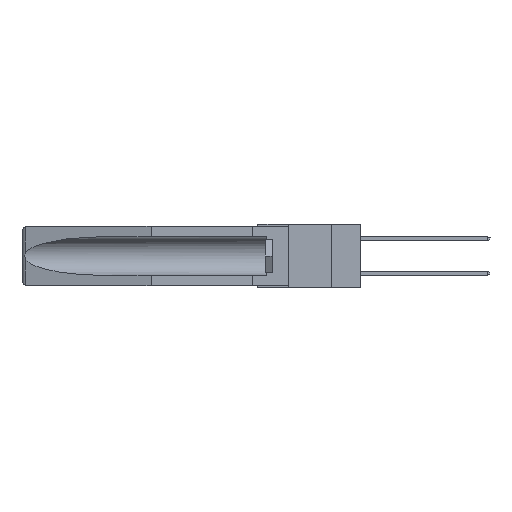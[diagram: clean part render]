
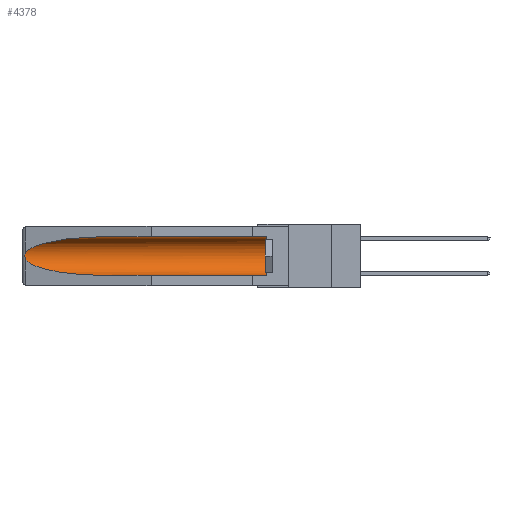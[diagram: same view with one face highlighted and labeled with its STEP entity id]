
A CAD part, left-side view. The second image highlights one B-rep face of the part: STEP entity #4378.
In plain terms, the highlighted cylindrical face has radius 2.857 mm (diameter 5.715 mm), a partial arc.
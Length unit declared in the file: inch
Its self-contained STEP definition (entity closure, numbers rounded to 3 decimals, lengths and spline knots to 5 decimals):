
#299 = EDGE_CURVE ( 'NONE', #5602, #23716, #3488, .T. ) ;
#722 = CARTESIAN_POINT ( 'NONE',  ( 0.155, 1.07973, -0.284 ) ) ;
#1227 = CARTESIAN_POINT ( 'NONE',  ( 0.25451, 1.48313, -0.09465 ) ) ;
#1373 = CARTESIAN_POINT ( 'NONE',  ( 0.155, 0.126, -0.1715 ) ) ;
#1454 = VECTOR ( 'NONE', #25289, 39.37008 ) ;
#3338 = ORIENTED_EDGE ( 'NONE', *, *, #299, .T. ) ;
#3488 = CIRCLE ( 'NONE', #10674, 0.1125 ) ;
#4350 = CARTESIAN_POINT ( 'NONE',  ( 0.25451, 1.48313, -0.24835 ) ) ;
#4378 = ADVANCED_FACE ( 'NONE', ( #20549 ), #23353, .F. ) ;
#4479 = EDGE_LOOP ( 'NONE', ( #23887, #13924, #23803, #11658, #3338, #22921 ) ) ;
#4938 = CARTESIAN_POINT ( 'NONE',  ( 0.155, -0.30754, -0.284 ) ) ;
#5281 = LINE ( 'NONE', #4938, #1454 ) ;
#5602 = VERTEX_POINT ( 'NONE', #13112 ) ;
#7306 = CARTESIAN_POINT ( 'NONE',  ( 0.155, 0.126, -0.059 ) ) ;
#7563 = CARTESIAN_POINT ( 'NONE',  ( 0.2675, 1.53308, -0.17534 ) ) ;
#7994 = CARTESIAN_POINT ( 'NONE',  ( 0.26537, 1.52718, -0.14972 ) ) ;
#9085 = CARTESIAN_POINT ( 'NONE',  ( 0.155, -0.30754, -0.059 ) ) ;
#9726 = CARTESIAN_POINT ( 'NONE',  ( 0.26654, 1.53092, -0.15636 ) ) ;
#10370 = CARTESIAN_POINT ( 'NONE',  ( 0.26537, 1.52718, -0.19328 ) ) ;
#10674 = AXIS2_PLACEMENT_3D ( 'NONE', #1373, #12687, #14983 ) ;
#11658 = ORIENTED_EDGE ( 'NONE', *, *, #19397, .F. ) ;
#12113 = CARTESIAN_POINT ( 'NONE',  ( 0.2673, 1.5327, -0.16383 ) ) ;
#12311 = VERTEX_POINT ( 'NONE', #10370 ) ;
#12448 = EDGE_CURVE ( 'NONE', #24427, #22170, #12963, .T. ) ;
#12450 = CARTESIAN_POINT ( 'NONE',  ( 0.21114, 1.30732, -0.059 ) ) ;
#12556 = LINE ( 'NONE', #9085, #17894 ) ;
#12687 = DIRECTION ( 'NONE',  ( 0., -1., 0. ) ) ;
#12963 =( BOUNDED_CURVE ( )  B_SPLINE_CURVE ( 3, ( #23489, #12450, #1227, #7994 ),
 .UNSPECIFIED., .F., .T. ) 
 B_SPLINE_CURVE_WITH_KNOTS ( ( 4, 4 ),
 ( 4.71239, 6.08839 ),
 .UNSPECIFIED. ) 
 CURVE ( )  GEOMETRIC_REPRESENTATION_ITEM ( )  RATIONAL_B_SPLINE_CURVE ( ( 1., 0.848, 0.848, 1. ) ) 
 REPRESENTATION_ITEM ( '' )  );
#13112 = CARTESIAN_POINT ( 'NONE',  ( 0.155, 0.126, -0.284 ) ) ;
#13924 = ORIENTED_EDGE ( 'NONE', *, *, #24759, .T. ) ;
#14204 = CARTESIAN_POINT ( 'NONE',  ( 0.26537, 1.52718, -0.14972 ) ) ;
#14936 = CARTESIAN_POINT ( 'NONE',  ( 0.155, 1.07973, -0.059 ) ) ;
#14983 = DIRECTION ( 'NONE',  ( 0., 0., 1. ) ) ;
#15290 = CARTESIAN_POINT ( 'NONE',  ( 0.26537, 1.52718, -0.19328 ) ) ;
#15914 = EDGE_CURVE ( 'NONE', #12311, #19764, #23066, .T. ) ;
#16440 = CARTESIAN_POINT ( 'NONE',  ( 0.26537, 1.52718, -0.14972 ) ) ;
#16891 = EDGE_CURVE ( 'NONE', #23716, #24427, #12556, .T. ) ;
#17748 = CARTESIAN_POINT ( 'NONE',  ( 0.21114, 1.30732, -0.284 ) ) ;
#17894 = VECTOR ( 'NONE', #24885, 39.37008 ) ;
#17946 = CARTESIAN_POINT ( 'NONE',  ( 0.26537, 1.52718, -0.19328 ) ) ;
#19397 = EDGE_CURVE ( 'NONE', #5602, #19764, #5281, .T. ) ;
#19764 = VERTEX_POINT ( 'NONE', #722 ) ;
#20452 = DIRECTION ( 'NONE',  ( 0., 0., 1. ) ) ;
#20549 = FACE_OUTER_BOUND ( 'NONE', #4479, .T. ) ;
#21108 = CARTESIAN_POINT ( 'NONE',  ( 0.2675, 1.53308, -0.16763 ) ) ;
#22170 = VERTEX_POINT ( 'NONE', #16440 ) ;
#22533 = CARTESIAN_POINT ( 'NONE',  ( 0.155, 1.07973, -0.284 ) ) ;
#22921 = ORIENTED_EDGE ( 'NONE', *, *, #16891, .T. ) ;
#23066 =( BOUNDED_CURVE ( )  B_SPLINE_CURVE ( 3, ( #17946, #4350, #17748, #22533 ),
 .UNSPECIFIED., .F., .F. ) 
 B_SPLINE_CURVE_WITH_KNOTS ( ( 4, 4 ),
 ( 0.1948, 1.5708 ),
 .UNSPECIFIED. ) 
 CURVE ( )  GEOMETRIC_REPRESENTATION_ITEM ( )  RATIONAL_B_SPLINE_CURVE ( ( 1., 0.848, 0.848, 1. ) ) 
 REPRESENTATION_ITEM ( '' )  );
#23251 = CARTESIAN_POINT ( 'NONE',  ( 0.26597, 1.52961, -0.15275 ) ) ;
#23353 = CYLINDRICAL_SURFACE ( 'NONE', #26988, 0.1125 ) ;
#23489 = CARTESIAN_POINT ( 'NONE',  ( 0.155, 1.07973, -0.059 ) ) ;
#23658 = CARTESIAN_POINT ( 'NONE',  ( 0.26597, 1.5296, -0.19026 ) ) ;
#23716 = VERTEX_POINT ( 'NONE', #7306 ) ;
#23803 = ORIENTED_EDGE ( 'NONE', *, *, #15914, .T. ) ;
#23887 = ORIENTED_EDGE ( 'NONE', *, *, #12448, .T. ) ;
#24427 = VERTEX_POINT ( 'NONE', #14936 ) ;
#24759 = EDGE_CURVE ( 'NONE', #22170, #12311, #25253, .T. ) ;
#24785 = CARTESIAN_POINT ( 'NONE',  ( 0.155, -0.30754, -0.1715 ) ) ;
#24885 = DIRECTION ( 'NONE',  ( 0., 1., 0. ) ) ;
#25253 = B_SPLINE_CURVE_WITH_KNOTS ( 'NONE', 3,
 ( #14204, #23251, #9726, #12113, #21108, #7563, #27856, #26200, #23658, #15290 ),
 .UNSPECIFIED., .F., .F.,
 ( 4, 2, 2, 2, 4 ),
 ( 0., 0.00029, 0.00058, 0.00087, 0.00117 ),
 .UNSPECIFIED. ) ;
#25289 = DIRECTION ( 'NONE',  ( 0., 1., 0. ) ) ;
#26200 = CARTESIAN_POINT ( 'NONE',  ( 0.26655, 1.53094, -0.18657 ) ) ;
#26988 = AXIS2_PLACEMENT_3D ( 'NONE', #24785, #27013, #20452 ) ;
#27013 = DIRECTION ( 'NONE',  ( 0., 1., 0. ) ) ;
#27856 = CARTESIAN_POINT ( 'NONE',  ( 0.2673, 1.53269, -0.17917 ) ) ;
